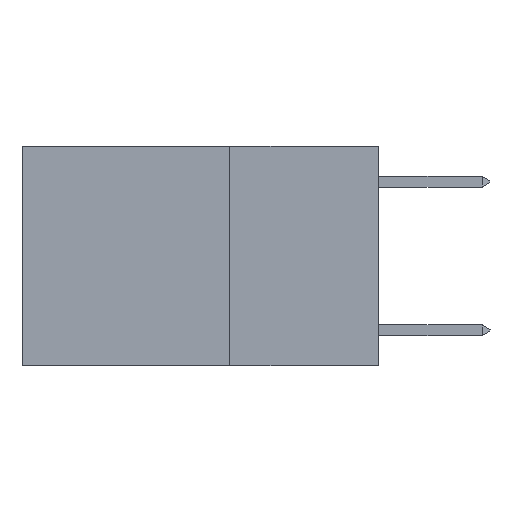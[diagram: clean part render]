
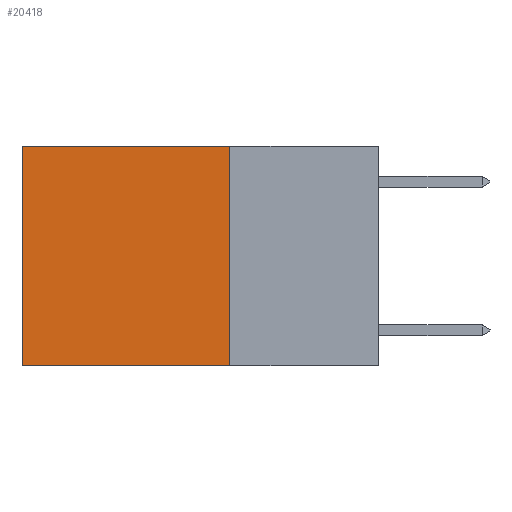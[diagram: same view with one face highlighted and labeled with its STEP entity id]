
A CAD part, left-side view. The second image highlights one B-rep face of the part: STEP entity #20418.
In plain terms, the highlighted planar face has unit normal (-1, 0, 0).
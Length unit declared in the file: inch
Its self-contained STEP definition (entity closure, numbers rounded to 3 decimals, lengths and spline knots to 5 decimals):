
#2657 = EDGE_CURVE ( 'NONE', #14012, #20447, #20748, .T. ) ;
#3946 = CARTESIAN_POINT ( 'NONE',  ( 0.2625, 0.25, -0.37 ) ) ;
#3956 = VECTOR ( 'NONE', #4648, 39.37008 ) ;
#3983 = LINE ( 'NONE', #4967, #3956 ) ;
#4648 = DIRECTION ( 'NONE',  ( 0., 0., -1. ) ) ;
#4967 = CARTESIAN_POINT ( 'NONE',  ( 0.2625, 0.6, 0. ) ) ;
#7703 = CARTESIAN_POINT ( 'NONE',  ( 0.2625, 0.6, -0.37 ) ) ;
#7906 = FACE_OUTER_BOUND ( 'NONE', #11379, .T. ) ;
#9182 = DIRECTION ( 'NONE',  ( 0., 0., -1. ) ) ;
#9261 = DIRECTION ( 'NONE',  ( 1., 0., 0. ) ) ;
#9264 = VERTEX_POINT ( 'NONE', #24494 ) ;
#9332 = CARTESIAN_POINT ( 'NONE',  ( 0.2625, 0.25, 0. ) ) ;
#9519 = PLANE ( 'NONE',  #9767 ) ;
#9721 = ORIENTED_EDGE ( 'NONE', *, *, #13989, .T. ) ;
#9767 = AXIS2_PLACEMENT_3D ( 'NONE', #9332, #9261, #9182 ) ;
#11379 = EDGE_LOOP ( 'NONE', ( #9721, #18489, #25571, #27577 ) ) ;
#11785 = EDGE_CURVE ( 'NONE', #12707, #14012, #20060, .T. ) ;
#12707 = VERTEX_POINT ( 'NONE', #27295 ) ;
#13082 = DIRECTION ( 'NONE',  ( 0., 1., 0. ) ) ;
#13266 = CARTESIAN_POINT ( 'NONE',  ( 0.2625, 0.25, 0. ) ) ;
#13989 = EDGE_CURVE ( 'NONE', #9264, #20447, #3983, .T. ) ;
#14012 = VERTEX_POINT ( 'NONE', #3946 ) ;
#14912 = DIRECTION ( 'NONE',  ( 0., 0., -1. ) ) ;
#15041 = CARTESIAN_POINT ( 'NONE',  ( 0.2625, 0.25, 0. ) ) ;
#18489 = ORIENTED_EDGE ( 'NONE', *, *, #2657, .F. ) ;
#20060 = LINE ( 'NONE', #15041, #20282 ) ;
#20282 = VECTOR ( 'NONE', #14912, 39.37008 ) ;
#20311 = VECTOR ( 'NONE', #13082, 39.37008 ) ;
#20418 = ADVANCED_FACE ( 'NONE', ( #7906 ), #9519, .F. ) ;
#20447 = VERTEX_POINT ( 'NONE', #7703 ) ;
#20636 = LINE ( 'NONE', #13266, #20311 ) ;
#20748 = LINE ( 'NONE', #26928, #23060 ) ;
#22452 = EDGE_CURVE ( 'NONE', #12707, #9264, #20636, .T. ) ;
#23060 = VECTOR ( 'NONE', #26904, 39.37008 ) ;
#24494 = CARTESIAN_POINT ( 'NONE',  ( 0.2625, 0.6, 0. ) ) ;
#25571 = ORIENTED_EDGE ( 'NONE', *, *, #11785, .F. ) ;
#26904 = DIRECTION ( 'NONE',  ( 0., 1., 0. ) ) ;
#26928 = CARTESIAN_POINT ( 'NONE',  ( 0.2625, 0.25, -0.37 ) ) ;
#27295 = CARTESIAN_POINT ( 'NONE',  ( 0.2625, 0.25, 0. ) ) ;
#27577 = ORIENTED_EDGE ( 'NONE', *, *, #22452, .T. ) ;
